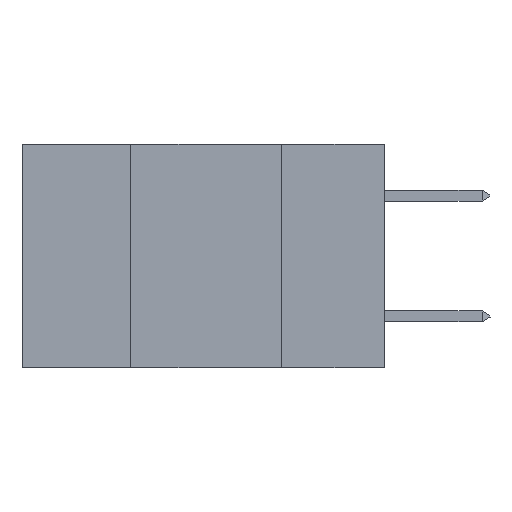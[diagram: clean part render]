
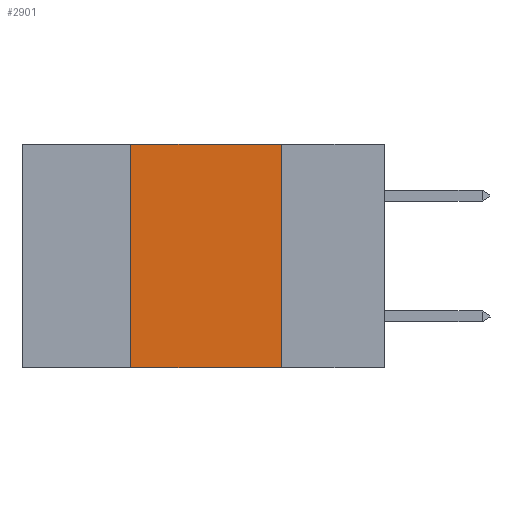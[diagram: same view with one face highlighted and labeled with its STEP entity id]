
A CAD part, left-side view. The second image highlights one B-rep face of the part: STEP entity #2901.
In plain terms, the highlighted planar face has unit normal (-1, 0, 0).
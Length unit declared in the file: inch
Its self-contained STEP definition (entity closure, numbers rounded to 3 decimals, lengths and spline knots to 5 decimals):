
#850 = CARTESIAN_POINT ( 'NONE',  ( 0., 0.6, 0. ) ) ;
#879 = CARTESIAN_POINT ( 'NONE',  ( 0., 0.42, -0.37 ) ) ;
#2668 = PLANE ( 'NONE',  #4965 ) ;
#2883 = CARTESIAN_POINT ( 'NONE',  ( 0., 0.6, -0.37 ) ) ;
#2901 = ADVANCED_FACE ( 'NONE', ( #6299 ), #2668, .F. ) ;
#3766 = CARTESIAN_POINT ( 'NONE',  ( 0., 0.42, 0. ) ) ;
#4125 = CARTESIAN_POINT ( 'NONE',  ( 0., 0.17, -0.37 ) ) ;
#4218 = ORIENTED_EDGE ( 'NONE', *, *, #14085, .F. ) ;
#4345 = VERTEX_POINT ( 'NONE', #879 ) ;
#4512 = VECTOR ( 'NONE', #10561, 39.37008 ) ;
#4562 = EDGE_LOOP ( 'NONE', ( #13134, #4218, #9611, #14549 ) ) ;
#4848 = LINE ( 'NONE', #5212, #12263 ) ;
#4965 = AXIS2_PLACEMENT_3D ( 'NONE', #9807, #10620, #7264 ) ;
#5212 = CARTESIAN_POINT ( 'NONE',  ( 0., 0.42, 0. ) ) ;
#5471 = VECTOR ( 'NONE', #11187, 39.37008 ) ;
#6299 = FACE_OUTER_BOUND ( 'NONE', #4562, .T. ) ;
#7264 = DIRECTION ( 'NONE',  ( 0., 0., -1. ) ) ;
#7581 = DIRECTION ( 'NONE',  ( 0., -1., 0. ) ) ;
#7816 = EDGE_CURVE ( 'NONE', #4345, #11412, #4848, .T. ) ;
#7859 = VERTEX_POINT ( 'NONE', #4125 ) ;
#8452 = EDGE_CURVE ( 'NONE', #9628, #7859, #13074, .T. ) ;
#9611 = ORIENTED_EDGE ( 'NONE', *, *, #7816, .F. ) ;
#9628 = VERTEX_POINT ( 'NONE', #14099 ) ;
#9807 = CARTESIAN_POINT ( 'NONE',  ( 0., 0.6, 0. ) ) ;
#10433 = EDGE_CURVE ( 'NONE', #4345, #7859, #13758, .T. ) ;
#10561 = DIRECTION ( 'NONE',  ( 0., -1., 0. ) ) ;
#10568 = LINE ( 'NONE', #850, #10739 ) ;
#10620 = DIRECTION ( 'NONE',  ( 1., 0., 0. ) ) ;
#10739 = VECTOR ( 'NONE', #7581, 39.37008 ) ;
#11187 = DIRECTION ( 'NONE',  ( 0., 0., -1. ) ) ;
#11412 = VERTEX_POINT ( 'NONE', #3766 ) ;
#12263 = VECTOR ( 'NONE', #13289, 39.37008 ) ;
#13074 = LINE ( 'NONE', #13513, #5471 ) ;
#13134 = ORIENTED_EDGE ( 'NONE', *, *, #8452, .F. ) ;
#13289 = DIRECTION ( 'NONE',  ( 0., 0., 1. ) ) ;
#13513 = CARTESIAN_POINT ( 'NONE',  ( 0., 0.17, 0. ) ) ;
#13758 = LINE ( 'NONE', #2883, #4512 ) ;
#14085 = EDGE_CURVE ( 'NONE', #11412, #9628, #10568, .T. ) ;
#14099 = CARTESIAN_POINT ( 'NONE',  ( 0., 0.17, 0. ) ) ;
#14549 = ORIENTED_EDGE ( 'NONE', *, *, #10433, .T. ) ;
